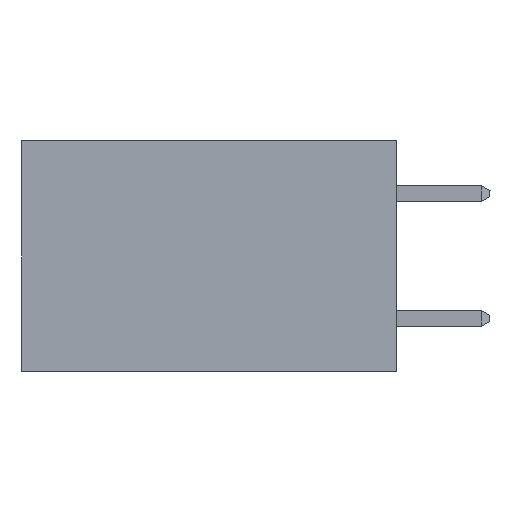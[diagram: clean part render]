
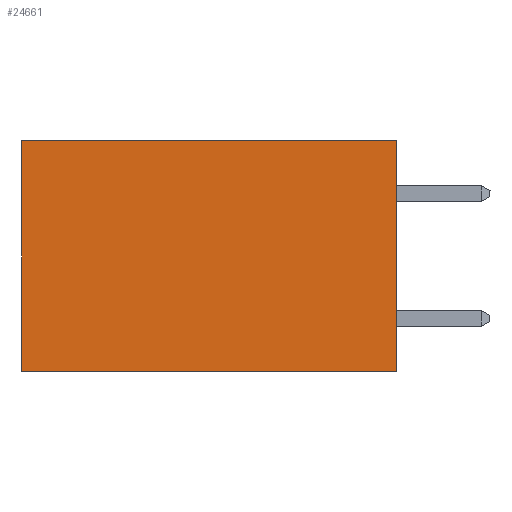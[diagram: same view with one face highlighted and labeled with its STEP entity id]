
A CAD part, left-side view. The second image highlights one B-rep face of the part: STEP entity #24661.
In plain terms, the highlighted planar face has unit normal (-1, 0, 0).
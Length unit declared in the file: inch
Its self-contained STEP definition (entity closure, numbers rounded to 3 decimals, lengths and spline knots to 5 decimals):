
#1081 = EDGE_LOOP ( 'NONE', ( #15054, #19765, #1572, #26264 ) ) ;
#1556 = DIRECTION ( 'NONE',  ( 0., 0., -1. ) ) ;
#1572 = ORIENTED_EDGE ( 'NONE', *, *, #23794, .F. ) ;
#3301 = CARTESIAN_POINT ( 'NONE',  ( 0.2615, 0.6, -0.37 ) ) ;
#3381 = VERTEX_POINT ( 'NONE', #7671 ) ;
#3536 = CARTESIAN_POINT ( 'NONE',  ( 0.2615, 0., -0.37 ) ) ;
#4598 = EDGE_CURVE ( 'NONE', #4689, #5001, #23087, .T. ) ;
#4689 = VERTEX_POINT ( 'NONE', #11217 ) ;
#4731 = FACE_OUTER_BOUND ( 'NONE', #1081, .T. ) ;
#4832 = VECTOR ( 'NONE', #14497, 39.37008 ) ;
#5001 = VERTEX_POINT ( 'NONE', #3301 ) ;
#7033 = VECTOR ( 'NONE', #12101, 39.37008 ) ;
#7428 = VERTEX_POINT ( 'NONE', #7926 ) ;
#7671 = CARTESIAN_POINT ( 'NONE',  ( 0.2615, 0., 0. ) ) ;
#7797 = DIRECTION ( 'NONE',  ( 0., 0., -1. ) ) ;
#7926 = CARTESIAN_POINT ( 'NONE',  ( 0.2615, 0., -0.37 ) ) ;
#8096 = AXIS2_PLACEMENT_3D ( 'NONE', #17762, #19792, #7797 ) ;
#9520 = LINE ( 'NONE', #20974, #13563 ) ;
#11217 = CARTESIAN_POINT ( 'NONE',  ( 0.2615, 0.6, 0. ) ) ;
#11220 = CARTESIAN_POINT ( 'NONE',  ( 0.2615, 0.6, -0.37 ) ) ;
#12101 = DIRECTION ( 'NONE',  ( 0., 0., -1. ) ) ;
#13563 = VECTOR ( 'NONE', #23029, 39.37008 ) ;
#14497 = DIRECTION ( 'NONE',  ( 0., 1., 0. ) ) ;
#14864 = VECTOR ( 'NONE', #1556, 39.37008 ) ;
#15054 = ORIENTED_EDGE ( 'NONE', *, *, #4598, .T. ) ;
#15500 = LINE ( 'NONE', #3536, #14864 ) ;
#16160 = LINE ( 'NONE', #16425, #4832 ) ;
#16425 = CARTESIAN_POINT ( 'NONE',  ( 0.2615, 0., 0. ) ) ;
#17762 = CARTESIAN_POINT ( 'NONE',  ( 0.2615, 0., -0.37 ) ) ;
#17839 = EDGE_CURVE ( 'NONE', #7428, #5001, #9520, .T. ) ;
#19765 = ORIENTED_EDGE ( 'NONE', *, *, #17839, .F. ) ;
#19792 = DIRECTION ( 'NONE',  ( 1., 0., 0. ) ) ;
#20974 = CARTESIAN_POINT ( 'NONE',  ( 0.2615, 0., -0.37 ) ) ;
#21355 = EDGE_CURVE ( 'NONE', #3381, #4689, #16160, .T. ) ;
#23029 = DIRECTION ( 'NONE',  ( 0., 1., 0. ) ) ;
#23087 = LINE ( 'NONE', #11220, #7033 ) ;
#23794 = EDGE_CURVE ( 'NONE', #3381, #7428, #15500, .T. ) ;
#23807 = PLANE ( 'NONE',  #8096 ) ;
#24661 = ADVANCED_FACE ( 'NONE', ( #4731 ), #23807, .F. ) ;
#26264 = ORIENTED_EDGE ( 'NONE', *, *, #21355, .T. ) ;
